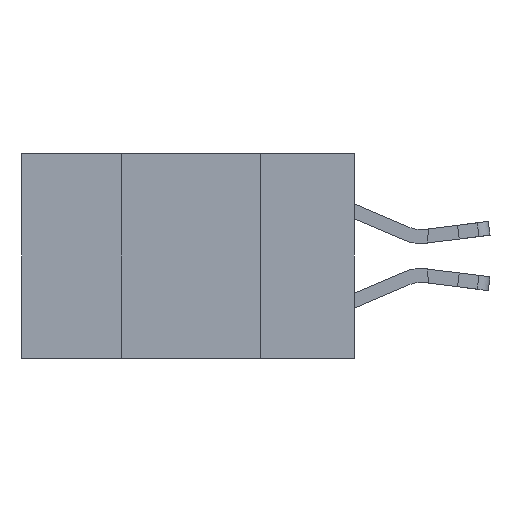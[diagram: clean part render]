
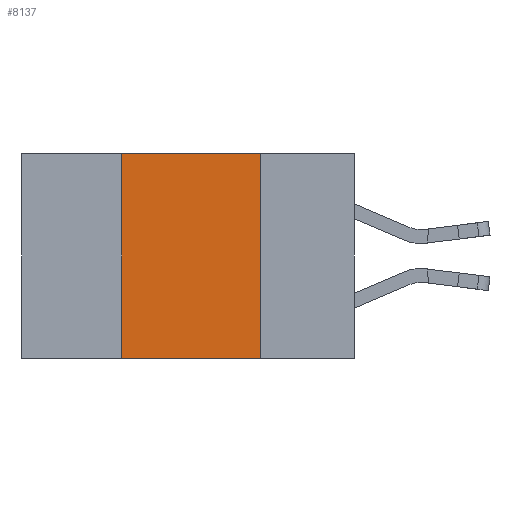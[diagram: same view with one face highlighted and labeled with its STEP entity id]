
A CAD part, left-side view. The second image highlights one B-rep face of the part: STEP entity #8137.
In plain terms, the highlighted planar face has unit normal (-1, 0, 0).
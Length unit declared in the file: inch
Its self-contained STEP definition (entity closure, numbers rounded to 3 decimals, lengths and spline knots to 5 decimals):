
#75 = DIRECTION ( 'NONE',  ( 0., -1., 0. ) ) ;
#175 = CARTESIAN_POINT ( 'NONE',  ( 0., 0.6, 0. ) ) ;
#1015 = CARTESIAN_POINT ( 'NONE',  ( 0., 0.17, -0.37 ) ) ;
#1442 = CARTESIAN_POINT ( 'NONE',  ( 0., 0.17, 0. ) ) ;
#1823 = LINE ( 'NONE', #2458, #8859 ) ;
#2458 = CARTESIAN_POINT ( 'NONE',  ( 0., 0.42, 0. ) ) ;
#2491 = EDGE_LOOP ( 'NONE', ( #4372, #6740, #11339, #11575 ) ) ;
#2792 = AXIS2_PLACEMENT_3D ( 'NONE', #175, #4090, #10304 ) ;
#3253 = VECTOR ( 'NONE', #7720, 39.37008 ) ;
#3537 = LINE ( 'NONE', #7737, #3253 ) ;
#3773 = EDGE_CURVE ( 'NONE', #7641, #7348, #9179, .T. ) ;
#3875 = EDGE_CURVE ( 'NONE', #10733, #7348, #3537, .T. ) ;
#4090 = DIRECTION ( 'NONE',  ( 1., 0., 0. ) ) ;
#4372 = ORIENTED_EDGE ( 'NONE', *, *, #3773, .F. ) ;
#4942 = VECTOR ( 'NONE', #75, 39.37008 ) ;
#5979 = EDGE_CURVE ( 'NONE', #10733, #10627, #1823, .T. ) ;
#6008 = CARTESIAN_POINT ( 'NONE',  ( 0., 0.42, -0.37 ) ) ;
#6416 = EDGE_CURVE ( 'NONE', #10627, #7641, #7310, .T. ) ;
#6740 = ORIENTED_EDGE ( 'NONE', *, *, #6416, .F. ) ;
#6820 = VECTOR ( 'NONE', #7958, 39.37008 ) ;
#7310 = LINE ( 'NONE', #7582, #4942 ) ;
#7348 = VERTEX_POINT ( 'NONE', #1015 ) ;
#7582 = CARTESIAN_POINT ( 'NONE',  ( 0., 0.6, 0. ) ) ;
#7641 = VERTEX_POINT ( 'NONE', #1442 ) ;
#7672 = PLANE ( 'NONE',  #2792 ) ;
#7720 = DIRECTION ( 'NONE',  ( 0., -1., 0. ) ) ;
#7737 = CARTESIAN_POINT ( 'NONE',  ( 0., 0.6, -0.37 ) ) ;
#7858 = FACE_OUTER_BOUND ( 'NONE', #2491, .T. ) ;
#7948 = DIRECTION ( 'NONE',  ( 0., 0., 1. ) ) ;
#7958 = DIRECTION ( 'NONE',  ( 0., 0., -1. ) ) ;
#8123 = CARTESIAN_POINT ( 'NONE',  ( 0., 0.17, 0. ) ) ;
#8137 = ADVANCED_FACE ( 'NONE', ( #7858 ), #7672, .F. ) ;
#8626 = CARTESIAN_POINT ( 'NONE',  ( 0., 0.42, 0. ) ) ;
#8859 = VECTOR ( 'NONE', #7948, 39.37008 ) ;
#9179 = LINE ( 'NONE', #8123, #6820 ) ;
#10304 = DIRECTION ( 'NONE',  ( 0., 0., -1. ) ) ;
#10627 = VERTEX_POINT ( 'NONE', #8626 ) ;
#10733 = VERTEX_POINT ( 'NONE', #6008 ) ;
#11339 = ORIENTED_EDGE ( 'NONE', *, *, #5979, .F. ) ;
#11575 = ORIENTED_EDGE ( 'NONE', *, *, #3875, .T. ) ;
